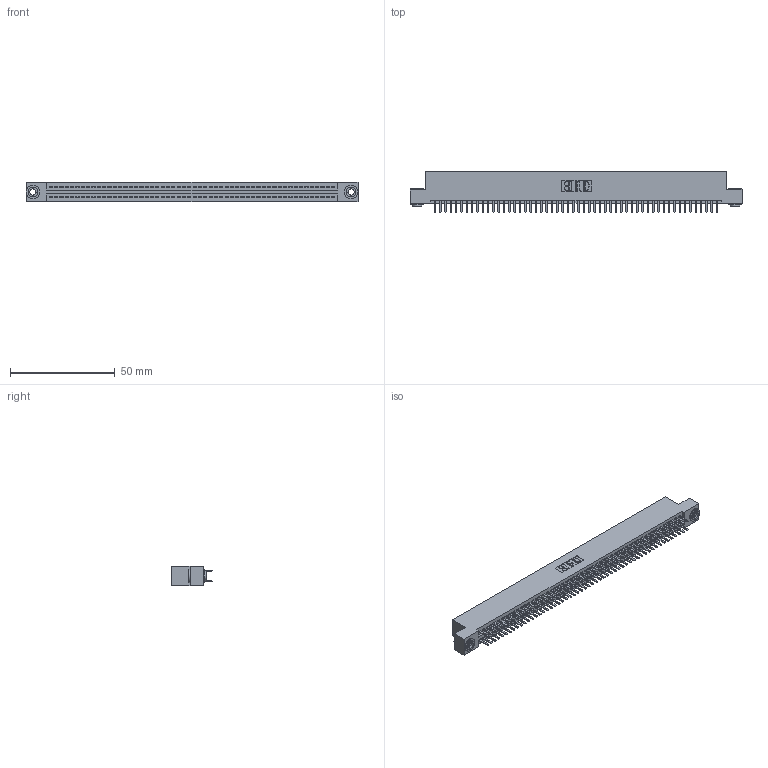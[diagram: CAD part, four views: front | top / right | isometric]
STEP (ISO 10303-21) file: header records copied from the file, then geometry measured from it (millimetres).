
FILE_DESCRIPTION (( 'STEP AP203' ), '1' );
FILE_NAME ('395-108-520-203.STEP', '2019-10-27T06:50:03', ( '' ), ( '' ), 'SwSTEP 2.0', 'SolidWorks 2016', '' );
FILE_SCHEMA (( 'CONFIG_CONTROL_DESIGN' ));
Length unit declared in the file: inch
Products named in the file (4): 345-292-001_345-293-120; 345-250-002_345-250-002-102; 395-108-520-203; 345 Part_Flush Mounting Lugs - 0.156 Dia-TH
Assembly tree (111 placements, depth 2):
  395-108-520-203
    345 Part_Flush Mounting Lugs - 0.156 Dia-TH
    345-292-001_345-293-120  x108
    345-250-002_345-250-002-102  x2
Bounding box: 158.37 x 19.68 x 9.4 mm (x, y, z)
Volume: 15467.4 mm3; surface area: 23199.8 mm2
Topology: 111 solids, 111 shells, 5996 faces, 17373 edges, 11290 vertices
Faces by surface type: plane 3870, cylinder 2118, cone 8
Entity records: 41518 total; most frequent: CARTESIAN_POINT 6935, ORIENTED_EDGE 6850, DIRECTION 6119, EDGE_CURVE 3425, VECTOR 3049, LINE 3049, VERTEX_POINT 2278, AXIS2_PLACEMENT_3D 1535
